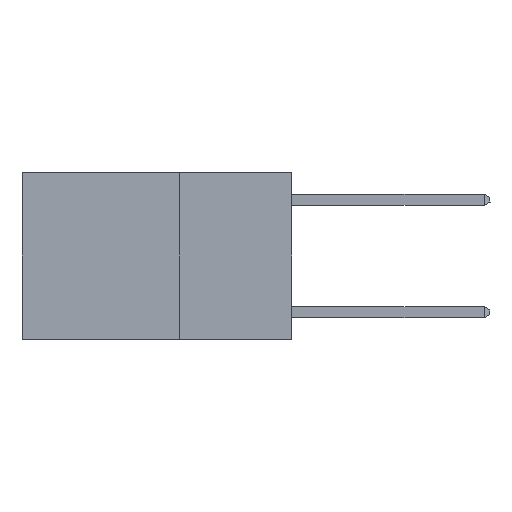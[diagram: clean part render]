
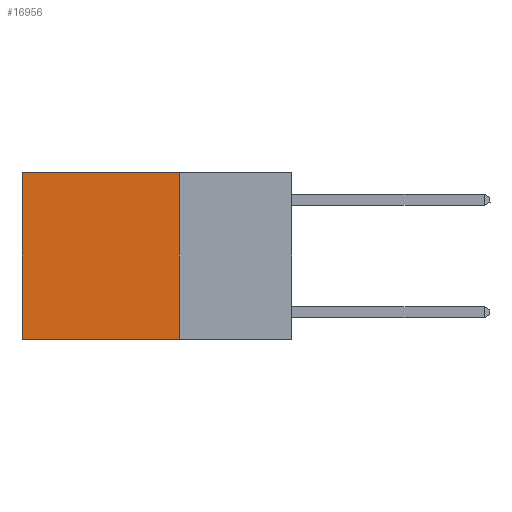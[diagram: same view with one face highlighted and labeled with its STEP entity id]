
A CAD part, left-side view. The second image highlights one B-rep face of the part: STEP entity #16956.
In plain terms, the highlighted planar face has unit normal (-1, 0, 0).
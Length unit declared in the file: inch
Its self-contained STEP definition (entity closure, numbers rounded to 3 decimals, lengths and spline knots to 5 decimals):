
#396 = CARTESIAN_POINT ( 'NONE',  ( 0.2625, 0.25, -0.37 ) ) ;
#791 = CARTESIAN_POINT ( 'NONE',  ( 0.2625, 0.25, 0. ) ) ;
#852 = VECTOR ( 'NONE', #898, 39.37008 ) ;
#898 = DIRECTION ( 'NONE',  ( 0., 0., -1. ) ) ;
#1602 = CARTESIAN_POINT ( 'NONE',  ( 0.2625, 0.6, -0.37 ) ) ;
#1630 = ORIENTED_EDGE ( 'NONE', *, *, #10314, .T. ) ;
#2105 = ORIENTED_EDGE ( 'NONE', *, *, #11885, .T. ) ;
#2257 = VERTEX_POINT ( 'NONE', #1602 ) ;
#2632 = CARTESIAN_POINT ( 'NONE',  ( 0.2625, 0.6, 0. ) ) ;
#2680 = VECTOR ( 'NONE', #9379, 39.37008 ) ;
#2770 = DIRECTION ( 'NONE',  ( 0., 0., -1. ) ) ;
#4034 = EDGE_CURVE ( 'NONE', #4375, #2257, #7354, .T. ) ;
#4375 = VERTEX_POINT ( 'NONE', #13713 ) ;
#5917 = DIRECTION ( 'NONE',  ( 0., 1., 0. ) ) ;
#7231 = VECTOR ( 'NONE', #5917, 39.37008 ) ;
#7354 = LINE ( 'NONE', #396, #7231 ) ;
#8909 = LINE ( 'NONE', #791, #13574 ) ;
#9102 = LINE ( 'NONE', #14834, #2680 ) ;
#9379 = DIRECTION ( 'NONE',  ( 0., 0., -1. ) ) ;
#9803 = CARTESIAN_POINT ( 'NONE',  ( 0.2625, 0.25, 0. ) ) ;
#10314 = EDGE_CURVE ( 'NONE', #14616, #2257, #13220, .T. ) ;
#10358 = DIRECTION ( 'NONE',  ( 0., 1., 0. ) ) ;
#11117 = AXIS2_PLACEMENT_3D ( 'NONE', #9803, #15080, #2770 ) ;
#11561 = EDGE_CURVE ( 'NONE', #13531, #4375, #9102, .T. ) ;
#11885 = EDGE_CURVE ( 'NONE', #13531, #14616, #8909, .T. ) ;
#11982 = CARTESIAN_POINT ( 'NONE',  ( 0.2625, 0.6, 0. ) ) ;
#12250 = ORIENTED_EDGE ( 'NONE', *, *, #11561, .F. ) ;
#13220 = LINE ( 'NONE', #11982, #852 ) ;
#13531 = VERTEX_POINT ( 'NONE', #13556 ) ;
#13556 = CARTESIAN_POINT ( 'NONE',  ( 0.2625, 0.25, 0. ) ) ;
#13574 = VECTOR ( 'NONE', #10358, 39.37008 ) ;
#13713 = CARTESIAN_POINT ( 'NONE',  ( 0.2625, 0.25, -0.37 ) ) ;
#14616 = VERTEX_POINT ( 'NONE', #2632 ) ;
#14834 = CARTESIAN_POINT ( 'NONE',  ( 0.2625, 0.25, 0. ) ) ;
#15080 = DIRECTION ( 'NONE',  ( 1., 0., 0. ) ) ;
#15248 = FACE_OUTER_BOUND ( 'NONE', #16511, .T. ) ;
#16312 = ORIENTED_EDGE ( 'NONE', *, *, #4034, .F. ) ;
#16511 = EDGE_LOOP ( 'NONE', ( #1630, #16312, #12250, #2105 ) ) ;
#16956 = ADVANCED_FACE ( 'NONE', ( #15248 ), #17586, .F. ) ;
#17586 = PLANE ( 'NONE',  #11117 ) ;
